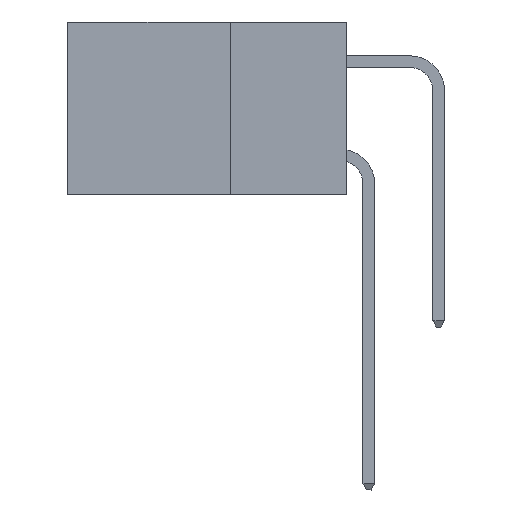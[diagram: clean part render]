
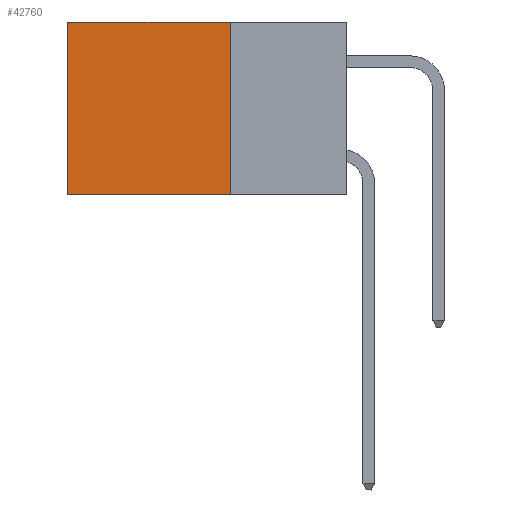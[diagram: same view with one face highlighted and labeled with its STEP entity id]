
A CAD part, left-side view. The second image highlights one B-rep face of the part: STEP entity #42760.
In plain terms, the highlighted planar face has unit normal (-1, 0, 0).
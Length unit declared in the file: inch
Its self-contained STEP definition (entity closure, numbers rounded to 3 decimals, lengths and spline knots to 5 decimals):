
#911 = DIRECTION ( 'NONE',  ( 0., 1., 0. ) ) ;
#1984 = DIRECTION ( 'NONE',  ( 0., 0., -1. ) ) ;
#2121 = PLANE ( 'NONE',  #6957 ) ;
#4001 = CARTESIAN_POINT ( 'NONE',  ( 0.2875, 0.6, -0.37 ) ) ;
#4807 = CARTESIAN_POINT ( 'NONE',  ( 0.2875, 0.6, 0. ) ) ;
#5098 = DIRECTION ( 'NONE',  ( 0., 0., -1. ) ) ;
#5425 = ORIENTED_EDGE ( 'NONE', *, *, #28369, .T. ) ;
#6278 = EDGE_CURVE ( 'NONE', #33226, #11385, #35530, .T. ) ;
#6835 = CARTESIAN_POINT ( 'NONE',  ( 0.2875, 0.25, 0. ) ) ;
#6957 = AXIS2_PLACEMENT_3D ( 'NONE', #22800, #26478, #1984 ) ;
#10340 = EDGE_LOOP ( 'NONE', ( #11805, #27401, #18980, #5425 ) ) ;
#11385 = VERTEX_POINT ( 'NONE', #4001 ) ;
#11805 = ORIENTED_EDGE ( 'NONE', *, *, #6278, .T. ) ;
#11955 = CARTESIAN_POINT ( 'NONE',  ( 0.2875, 0.6, 0. ) ) ;
#11962 = CARTESIAN_POINT ( 'NONE',  ( 0.2875, 0.25, 0. ) ) ;
#12840 = VECTOR ( 'NONE', #911, 39.37008 ) ;
#12973 = VECTOR ( 'NONE', #29453, 39.37008 ) ;
#14906 = EDGE_CURVE ( 'NONE', #44867, #43458, #28766, .T. ) ;
#16233 = EDGE_CURVE ( 'NONE', #43458, #11385, #29160, .T. ) ;
#16750 = DIRECTION ( 'NONE',  ( 0., 1., 0. ) ) ;
#17006 = FACE_OUTER_BOUND ( 'NONE', #10340, .T. ) ;
#18980 = ORIENTED_EDGE ( 'NONE', *, *, #14906, .F. ) ;
#22326 = CARTESIAN_POINT ( 'NONE',  ( 0.2875, 0.25, -0.37 ) ) ;
#22789 = CARTESIAN_POINT ( 'NONE',  ( 0.2875, 0.25, 0. ) ) ;
#22800 = CARTESIAN_POINT ( 'NONE',  ( 0.2875, 0.25, 0. ) ) ;
#25759 = VECTOR ( 'NONE', #5098, 39.37008 ) ;
#26478 = DIRECTION ( 'NONE',  ( 1., 0., 0. ) ) ;
#27401 = ORIENTED_EDGE ( 'NONE', *, *, #16233, .F. ) ;
#28369 = EDGE_CURVE ( 'NONE', #44867, #33226, #40897, .T. ) ;
#28766 = LINE ( 'NONE', #11962, #12973 ) ;
#29160 = LINE ( 'NONE', #22326, #12840 ) ;
#29453 = DIRECTION ( 'NONE',  ( 0., 0., -1. ) ) ;
#31671 = VECTOR ( 'NONE', #16750, 39.37008 ) ;
#33226 = VERTEX_POINT ( 'NONE', #4807 ) ;
#35530 = LINE ( 'NONE', #11955, #25759 ) ;
#36442 = CARTESIAN_POINT ( 'NONE',  ( 0.2875, 0.25, -0.37 ) ) ;
#40897 = LINE ( 'NONE', #6835, #31671 ) ;
#42760 = ADVANCED_FACE ( 'NONE', ( #17006 ), #2121, .F. ) ;
#43458 = VERTEX_POINT ( 'NONE', #36442 ) ;
#44867 = VERTEX_POINT ( 'NONE', #22789 ) ;
